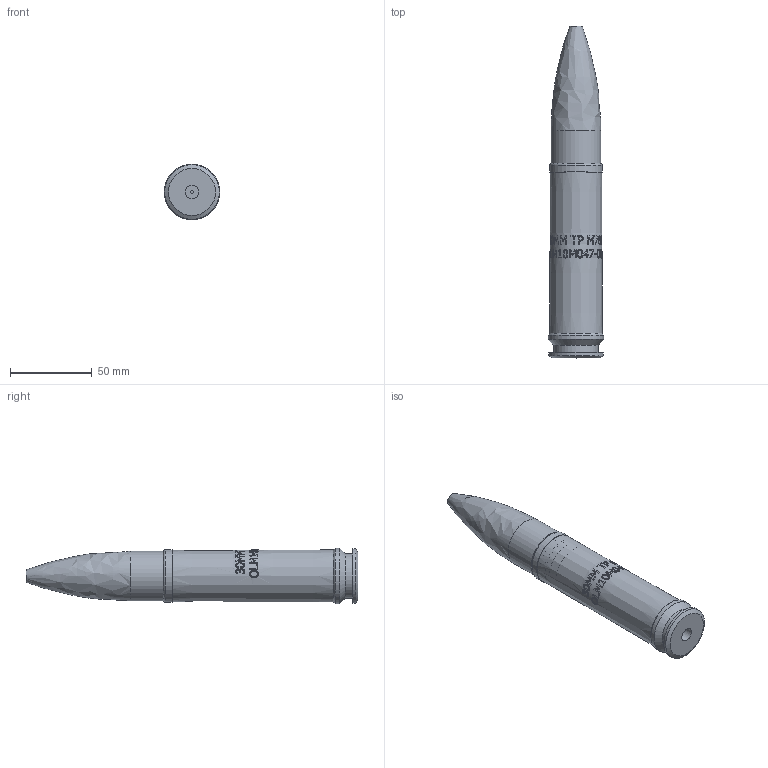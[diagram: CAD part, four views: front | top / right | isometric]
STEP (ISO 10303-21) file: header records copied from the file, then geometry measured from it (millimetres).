
FILE_DESCRIPTION((''),'2;1');
FILE_NAME('30mm GAU.stp','2012-12-04T12:09:17',('agarrett'),(''),'Autodesk Inventor 2012','Autodesk Inventor 2012','');
FILE_SCHEMA(('AUTOMOTIVE_DESIGN { 1 0 10303 214 1 1 1 1 }'));
Length unit declared in the file: inch
Products named in the file (3): 30mm GAU; 30mm Casing; 30_mm_Bullet
Assembly tree (2 placements, depth 2):
  30mm GAU
    30mm Casing
    30_mm_Bullet
Bounding box: 33.88 x 202.63 x 33.88 mm (x, y, z)
Volume: 74622.2 mm3; surface area: 33045.8 mm2
Topology: 2 solids, 2 shells, 66 faces, 346 edges, 324 vertices
Faces by surface type: cone 40, cylinder 11, plane 9, torus 4, sphere 1, bspline 1
Full cylindrical faces by diameter (mm): 1.778 x1, 3.353 x1, 8.382 x1, 26.975 x1, 30.378 x4, 32.004 x1, 33.35 x1, 33.884 x1
Entity records: 22687 total; most frequent: CARTESIAN_POINT 20205, ORIENTED_EDGE 644, VERTEX_POINT 322, EDGE_CURVE 322, B_SPLINE_CURVE_WITH_KNOTS 279, DIRECTION 223, EDGE_LOOP 130, AXIS2_PLACEMENT_3D 110
